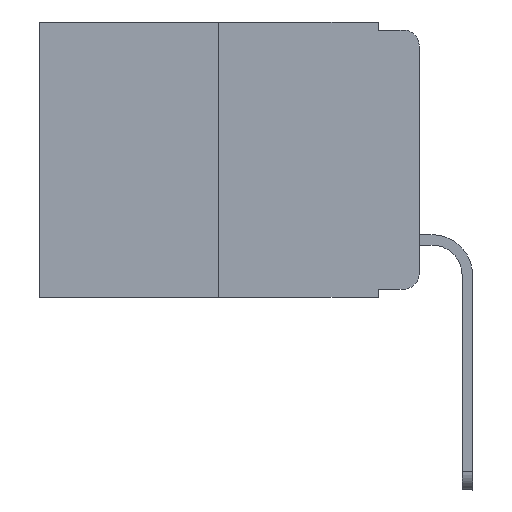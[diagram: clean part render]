
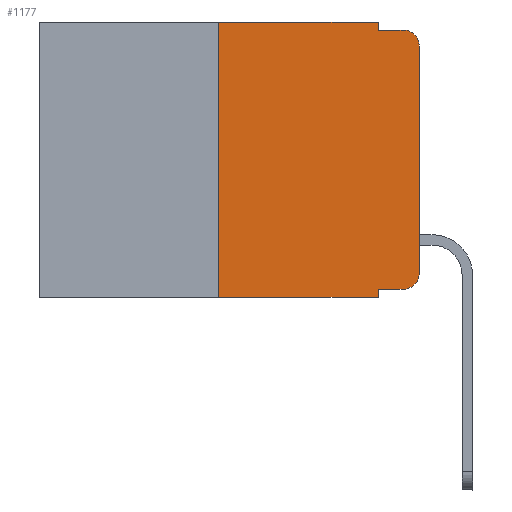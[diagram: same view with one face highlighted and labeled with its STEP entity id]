
A CAD part, left-side view. The second image highlights one B-rep face of the part: STEP entity #1177.
In plain terms, the highlighted planar face has unit normal (-1, 0, 0).
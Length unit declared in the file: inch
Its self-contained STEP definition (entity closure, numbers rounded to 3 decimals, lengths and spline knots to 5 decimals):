
#258 = CARTESIAN_POINT ( 'NONE',  ( 0., 0.051, -0.01 ) ) ;
#922 = VERTEX_POINT ( 'NONE', #18663 ) ;
#1177 = ADVANCED_FACE ( 'NONE', ( #12384 ), #5992, .F. ) ;
#1745 = LINE ( 'NONE', #258, #11732 ) ;
#2296 = CARTESIAN_POINT ( 'NONE',  ( 0., 0.02, -0.01 ) ) ;
#2622 = ORIENTED_EDGE ( 'NONE', *, *, #13593, .T. ) ;
#2849 = CARTESIAN_POINT ( 'NONE',  ( 0., 0.051, -0.01 ) ) ;
#2860 = ORIENTED_EDGE ( 'NONE', *, *, #15283, .T. ) ;
#3205 = VECTOR ( 'NONE', #4130, 39.37008 ) ;
#3239 = VERTEX_POINT ( 'NONE', #17117 ) ;
#3528 = DIRECTION ( 'NONE',  ( -1., 0., 0. ) ) ;
#3586 = CARTESIAN_POINT ( 'NONE',  ( 0., 0., -0.03 ) ) ;
#3649 = VERTEX_POINT ( 'NONE', #18648 ) ;
#3898 = CARTESIAN_POINT ( 'NONE',  ( 0., 0.473, -0.343 ) ) ;
#4130 = DIRECTION ( 'NONE',  ( 0., 0., 1. ) ) ;
#4514 = LINE ( 'NONE', #16981, #11245 ) ;
#4569 = EDGE_CURVE ( 'NONE', #4937, #8887, #19183, .T. ) ;
#4887 = CARTESIAN_POINT ( 'NONE',  ( 0., 0.02, -0.03 ) ) ;
#4937 = VERTEX_POINT ( 'NONE', #18389 ) ;
#4940 = CARTESIAN_POINT ( 'NONE',  ( 0., 0.02, -0.313 ) ) ;
#5109 = DIRECTION ( 'NONE',  ( 0., 0., 1. ) ) ;
#5505 = VECTOR ( 'NONE', #8295, 39.37008 ) ;
#5560 = VERTEX_POINT ( 'NONE', #6636 ) ;
#5992 = PLANE ( 'NONE',  #9431 ) ;
#6353 = CARTESIAN_POINT ( 'NONE',  ( 0., 0.473, 0. ) ) ;
#6636 = CARTESIAN_POINT ( 'NONE',  ( 0., 0.02, -0.333 ) ) ;
#6758 = ORIENTED_EDGE ( 'NONE', *, *, #8460, .F. ) ;
#6970 = ORIENTED_EDGE ( 'NONE', *, *, #13400, .F. ) ;
#7870 = VERTEX_POINT ( 'NONE', #15147 ) ;
#7908 = CIRCLE ( 'NONE', #19036, 0.02 ) ;
#8005 = LINE ( 'NONE', #12595, #9014 ) ;
#8006 = EDGE_CURVE ( 'NONE', #3239, #3649, #16849, .T. ) ;
#8292 = CARTESIAN_POINT ( 'NONE',  ( 0., 0.051, 0. ) ) ;
#8295 = DIRECTION ( 'NONE',  ( 0., -1., 0. ) ) ;
#8397 = VERTEX_POINT ( 'NONE', #12435 ) ;
#8460 = EDGE_CURVE ( 'NONE', #9552, #19075, #1745, .T. ) ;
#8887 = VERTEX_POINT ( 'NONE', #3586 ) ;
#9014 = VECTOR ( 'NONE', #11099, 39.37008 ) ;
#9388 = ORIENTED_EDGE ( 'NONE', *, *, #13451, .F. ) ;
#9431 = AXIS2_PLACEMENT_3D ( 'NONE', #13784, #15076, #12096 ) ;
#9547 = ORIENTED_EDGE ( 'NONE', *, *, #8006, .F. ) ;
#9552 = VERTEX_POINT ( 'NONE', #2849 ) ;
#9936 = CARTESIAN_POINT ( 'NONE',  ( 0., 0., 0. ) ) ;
#11099 = DIRECTION ( 'NONE',  ( 0., 0., -1. ) ) ;
#11245 = VECTOR ( 'NONE', #5109, 39.37008 ) ;
#11732 = VECTOR ( 'NONE', #13741, 39.37008 ) ;
#11773 = CARTESIAN_POINT ( 'NONE',  ( 0., 0.051, -0.333 ) ) ;
#12087 = EDGE_LOOP ( 'NONE', ( #15628, #19629, #6758, #9388, #9547, #6970, #2622, #17888, #2860, #12601 ) ) ;
#12096 = DIRECTION ( 'NONE',  ( 0., 0., -1. ) ) ;
#12339 = EDGE_CURVE ( 'NONE', #922, #8397, #15963, .T. ) ;
#12384 = FACE_OUTER_BOUND ( 'NONE', #12087, .T. ) ;
#12435 = CARTESIAN_POINT ( 'NONE',  ( 0., 0.051, -0.343 ) ) ;
#12595 = CARTESIAN_POINT ( 'NONE',  ( 0., 0.051, 0. ) ) ;
#12601 = ORIENTED_EDGE ( 'NONE', *, *, #13000, .T. ) ;
#13000 = EDGE_CURVE ( 'NONE', #5560, #4937, #7908, .T. ) ;
#13271 = LINE ( 'NONE', #11773, #16354 ) ;
#13282 = LINE ( 'NONE', #3898, #5505 ) ;
#13400 = EDGE_CURVE ( 'NONE', #7870, #3239, #4514, .T. ) ;
#13451 = EDGE_CURVE ( 'NONE', #3649, #9552, #8005, .T. ) ;
#13593 = EDGE_CURVE ( 'NONE', #7870, #8397, #13282, .T. ) ;
#13628 = VECTOR ( 'NONE', #17562, 39.37008 ) ;
#13669 = DIRECTION ( 'NONE',  ( 0., -1., 0. ) ) ;
#13741 = DIRECTION ( 'NONE',  ( 0., -1., 0. ) ) ;
#13784 = CARTESIAN_POINT ( 'NONE',  ( 0., 0.473, 0. ) ) ;
#13852 = EDGE_CURVE ( 'NONE', #8887, #19075, #18881, .T. ) ;
#15076 = DIRECTION ( 'NONE',  ( 1., 0., 0. ) ) ;
#15147 = CARTESIAN_POINT ( 'NONE',  ( 0., 0.25, -0.343 ) ) ;
#15283 = EDGE_CURVE ( 'NONE', #922, #5560, #13271, .T. ) ;
#15500 = DIRECTION ( 'NONE',  ( 0., 0., -1. ) ) ;
#15628 = ORIENTED_EDGE ( 'NONE', *, *, #4569, .T. ) ;
#15653 = DIRECTION ( 'NONE',  ( -1., 0., 0. ) ) ;
#15963 = LINE ( 'NONE', #8292, #13628 ) ;
#16339 = AXIS2_PLACEMENT_3D ( 'NONE', #4887, #15653, #17056 ) ;
#16354 = VECTOR ( 'NONE', #17843, 39.37008 ) ;
#16849 = LINE ( 'NONE', #6353, #19346 ) ;
#16981 = CARTESIAN_POINT ( 'NONE',  ( 0., 0.25, 0. ) ) ;
#17056 = DIRECTION ( 'NONE',  ( 0., 0., -1. ) ) ;
#17117 = CARTESIAN_POINT ( 'NONE',  ( 0., 0.25, 0. ) ) ;
#17562 = DIRECTION ( 'NONE',  ( 0., 0., -1. ) ) ;
#17843 = DIRECTION ( 'NONE',  ( 0., -1., 0. ) ) ;
#17888 = ORIENTED_EDGE ( 'NONE', *, *, #12339, .F. ) ;
#18389 = CARTESIAN_POINT ( 'NONE',  ( 0., 0., -0.313 ) ) ;
#18648 = CARTESIAN_POINT ( 'NONE',  ( 0., 0.051, 0. ) ) ;
#18663 = CARTESIAN_POINT ( 'NONE',  ( 0., 0.051, -0.333 ) ) ;
#18881 = CIRCLE ( 'NONE', #16339, 0.02 ) ;
#19036 = AXIS2_PLACEMENT_3D ( 'NONE', #4940, #3528, #15500 ) ;
#19075 = VERTEX_POINT ( 'NONE', #2296 ) ;
#19183 = LINE ( 'NONE', #9936, #3205 ) ;
#19346 = VECTOR ( 'NONE', #13669, 39.37008 ) ;
#19629 = ORIENTED_EDGE ( 'NONE', *, *, #13852, .T. ) ;
